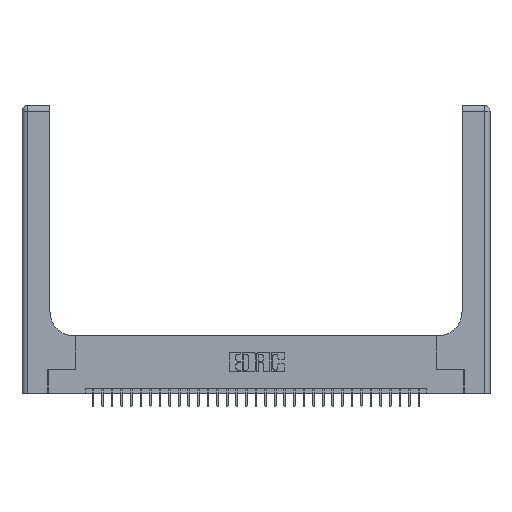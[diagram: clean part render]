
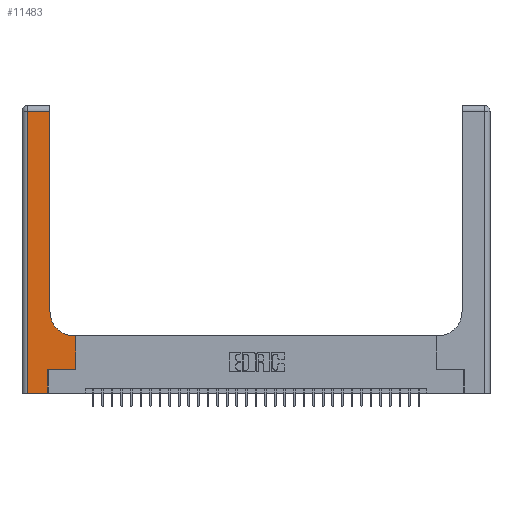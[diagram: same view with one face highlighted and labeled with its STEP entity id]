
A CAD part, top view. The second image highlights one B-rep face of the part: STEP entity #11483.
In plain terms, the highlighted planar face has unit normal (0, 0, 1).
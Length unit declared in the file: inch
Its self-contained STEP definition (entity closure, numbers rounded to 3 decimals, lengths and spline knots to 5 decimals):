
#319 = DIRECTION ( 'NONE',  ( -1., 0., 0. ) ) ;
#355 = DIRECTION ( 'NONE',  ( -1., 0., 0. ) ) ;
#774 = DIRECTION ( 'NONE',  ( 0., 1., 0. ) ) ;
#876 = DIRECTION ( 'NONE',  ( -1., 0., 0. ) ) ;
#1045 = VERTEX_POINT ( 'NONE', #11513 ) ;
#1153 = VERTEX_POINT ( 'NONE', #21590 ) ;
#1240 = LINE ( 'NONE', #19305, #5301 ) ;
#5301 = VECTOR ( 'NONE', #30351, 39.37008 ) ;
#5370 = VECTOR ( 'NONE', #15558, 39.37008 ) ;
#5567 = CARTESIAN_POINT ( 'NONE',  ( 0.5585, 0.25, 0.37 ) ) ;
#5776 = CARTESIAN_POINT ( 'NONE',  ( 0., 2.94, 0.37 ) ) ;
#6194 = EDGE_CURVE ( 'NONE', #1045, #9695, #23248, .T. ) ;
#7879 = CARTESIAN_POINT ( 'NONE',  ( 0., 3., 0.37 ) ) ;
#8120 = DIRECTION ( 'NONE',  ( 0., 1., 0. ) ) ;
#8202 = PLANE ( 'NONE',  #8575 ) ;
#8365 = EDGE_CURVE ( 'NONE', #29628, #12574, #29599, .T. ) ;
#8575 = AXIS2_PLACEMENT_3D ( 'NONE', #7879, #28799, #355 ) ;
#8808 = ORIENTED_EDGE ( 'NONE', *, *, #8365, .T. ) ;
#9137 = EDGE_CURVE ( 'NONE', #12735, #11776, #33182, .T. ) ;
#9695 = VERTEX_POINT ( 'NONE', #21621 ) ;
#9847 = DIRECTION ( 'NONE',  ( 0., -1., 0. ) ) ;
#9946 = VERTEX_POINT ( 'NONE', #13225 ) ;
#10252 = DIRECTION ( 'NONE',  ( 0., 0., -1. ) ) ;
#10498 = CARTESIAN_POINT ( 'NONE',  ( 0.2915, 3., 0.37 ) ) ;
#10711 = ORIENTED_EDGE ( 'NONE', *, *, #14960, .T. ) ;
#10848 = DIRECTION ( 'NONE',  ( 1., 0., 0. ) ) ;
#11136 = ORIENTED_EDGE ( 'NONE', *, *, #22025, .T. ) ;
#11483 = ADVANCED_FACE ( 'NONE', ( #18449 ), #8202, .F. ) ;
#11513 = CARTESIAN_POINT ( 'NONE',  ( 0.269, 0.25, 0.37 ) ) ;
#11776 = VERTEX_POINT ( 'NONE', #25226 ) ;
#12574 = VERTEX_POINT ( 'NONE', #27976 ) ;
#12735 = VERTEX_POINT ( 'NONE', #23869 ) ;
#12976 = DIRECTION ( 'NONE',  ( 1., 0., 0. ) ) ;
#13225 = CARTESIAN_POINT ( 'NONE',  ( 0.5585, 0.6, 0.37 ) ) ;
#13407 = LINE ( 'NONE', #16477, #24590 ) ;
#14062 = CARTESIAN_POINT ( 'NONE',  ( 0.06, 0., 0.37 ) ) ;
#14923 = VECTOR ( 'NONE', #9847, 39.37008 ) ;
#14960 = EDGE_CURVE ( 'NONE', #1153, #1045, #1240, .T. ) ;
#15197 = VECTOR ( 'NONE', #8120, 39.37008 ) ;
#15558 = DIRECTION ( 'NONE',  ( 1., 0., 0. ) ) ;
#15690 = ORIENTED_EDGE ( 'NONE', *, *, #31554, .T. ) ;
#16477 = CARTESIAN_POINT ( 'NONE',  ( 0., 0., 0.37 ) ) ;
#16558 = VECTOR ( 'NONE', #876, 39.37008 ) ;
#17507 = EDGE_CURVE ( 'NONE', #11776, #29628, #23463, .T. ) ;
#17937 = AXIS2_PLACEMENT_3D ( 'NONE', #31371, #10252, #12976 ) ;
#18449 = FACE_OUTER_BOUND ( 'NONE', #32872, .T. ) ;
#18526 = LINE ( 'NONE', #5567, #19593 ) ;
#19305 = CARTESIAN_POINT ( 'NONE',  ( 0.269, 0., 0.37 ) ) ;
#19593 = VECTOR ( 'NONE', #774, 39.37008 ) ;
#19881 = ORIENTED_EDGE ( 'NONE', *, *, #6194, .T. ) ;
#20831 = ORIENTED_EDGE ( 'NONE', *, *, #9137, .T. ) ;
#21590 = CARTESIAN_POINT ( 'NONE',  ( 0.269, 0., 0.37 ) ) ;
#21621 = CARTESIAN_POINT ( 'NONE',  ( 0.5585, 0.25, 0.37 ) ) ;
#22025 = EDGE_CURVE ( 'NONE', #26795, #1153, #13407, .T. ) ;
#22803 = LINE ( 'NONE', #33379, #14923 ) ;
#23248 = LINE ( 'NONE', #26281, #5370 ) ;
#23463 = LINE ( 'NONE', #10498, #15197 ) ;
#23869 = CARTESIAN_POINT ( 'NONE',  ( 0.5415, 0.6, 0.37 ) ) ;
#23872 = LINE ( 'NONE', #31543, #16558 ) ;
#24590 = VECTOR ( 'NONE', #10848, 39.37008 ) ;
#25226 = CARTESIAN_POINT ( 'NONE',  ( 0.2915, 0.85, 0.37 ) ) ;
#25339 = EDGE_CURVE ( 'NONE', #9946, #12735, #23872, .T. ) ;
#25498 = EDGE_CURVE ( 'NONE', #12574, #26795, #22803, .T. ) ;
#25526 = VECTOR ( 'NONE', #319, 39.37008 ) ;
#26105 = ORIENTED_EDGE ( 'NONE', *, *, #25498, .T. ) ;
#26281 = CARTESIAN_POINT ( 'NONE',  ( 0.269, 0.25, 0.37 ) ) ;
#26795 = VERTEX_POINT ( 'NONE', #14062 ) ;
#27976 = CARTESIAN_POINT ( 'NONE',  ( 0.06, 2.94, 0.37 ) ) ;
#28799 = DIRECTION ( 'NONE',  ( 0., 0., -1. ) ) ;
#29599 = LINE ( 'NONE', #5776, #25526 ) ;
#29628 = VERTEX_POINT ( 'NONE', #32635 ) ;
#30351 = DIRECTION ( 'NONE',  ( 0., 1., 0. ) ) ;
#31025 = ORIENTED_EDGE ( 'NONE', *, *, #17507, .T. ) ;
#31371 = CARTESIAN_POINT ( 'NONE',  ( 0.5415, 0.85, 0.37 ) ) ;
#31543 = CARTESIAN_POINT ( 'NONE',  ( 0.2915, 0.6, 0.37 ) ) ;
#31554 = EDGE_CURVE ( 'NONE', #9695, #9946, #18526, .T. ) ;
#31927 = ORIENTED_EDGE ( 'NONE', *, *, #25339, .T. ) ;
#32635 = CARTESIAN_POINT ( 'NONE',  ( 0.2915, 2.94, 0.37 ) ) ;
#32872 = EDGE_LOOP ( 'NONE', ( #31025, #8808, #26105, #11136, #10711, #19881, #15690, #31927, #20831 ) ) ;
#33182 = CIRCLE ( 'NONE', #17937, 0.25 ) ;
#33379 = CARTESIAN_POINT ( 'NONE',  ( 0.06, 3., 0.37 ) ) ;
